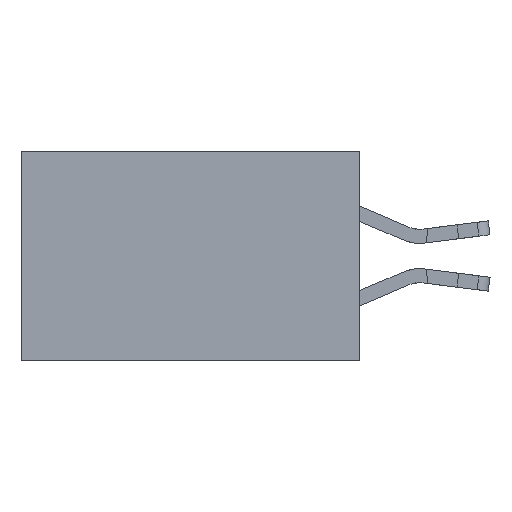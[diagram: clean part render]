
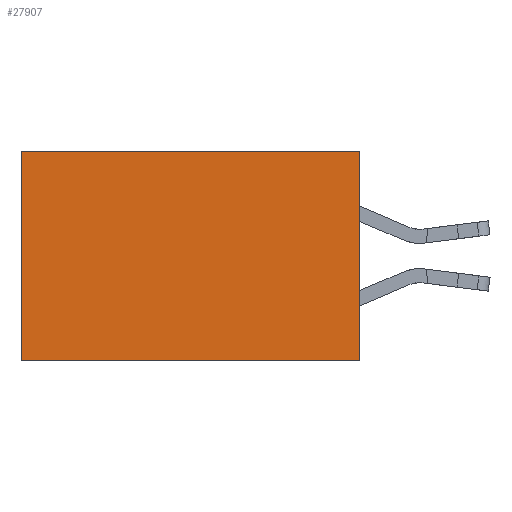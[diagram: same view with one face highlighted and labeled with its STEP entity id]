
A CAD part, left-side view. The second image highlights one B-rep face of the part: STEP entity #27907.
In plain terms, the highlighted planar face has unit normal (-1, 0, 0).
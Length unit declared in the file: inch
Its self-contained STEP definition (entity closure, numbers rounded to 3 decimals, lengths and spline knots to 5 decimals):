
#1503 = LINE ( 'NONE', #11780, #20072 ) ;
#2310 = DIRECTION ( 'NONE',  ( 0., 0., -1. ) ) ;
#2759 = DIRECTION ( 'NONE',  ( 0., 1., 0. ) ) ;
#4260 = EDGE_CURVE ( 'NONE', #8059, #28060, #25768, .T. ) ;
#5155 = ORIENTED_EDGE ( 'NONE', *, *, #7710, .T. ) ;
#6000 = CARTESIAN_POINT ( 'NONE',  ( 0.2875, 0., 0. ) ) ;
#6197 = PLANE ( 'NONE',  #6389 ) ;
#6389 = AXIS2_PLACEMENT_3D ( 'NONE', #13120, #17551, #21602 ) ;
#6698 = DIRECTION ( 'NONE',  ( 0., 0., -1. ) ) ;
#7710 = EDGE_CURVE ( 'NONE', #8059, #13851, #1503, .T. ) ;
#8059 = VERTEX_POINT ( 'NONE', #6000 ) ;
#10373 = ORIENTED_EDGE ( 'NONE', *, *, #21072, .T. ) ;
#10885 = VECTOR ( 'NONE', #6698, 39.37008 ) ;
#10946 = CARTESIAN_POINT ( 'NONE',  ( 0.2875, 0.6, 0. ) ) ;
#11146 = CARTESIAN_POINT ( 'NONE',  ( 0.2875, 0., 0. ) ) ;
#11780 = CARTESIAN_POINT ( 'NONE',  ( 0.2875, 0., 0. ) ) ;
#13120 = CARTESIAN_POINT ( 'NONE',  ( 0.2875, 0., 0. ) ) ;
#13851 = VERTEX_POINT ( 'NONE', #23755 ) ;
#14451 = CARTESIAN_POINT ( 'NONE',  ( 0.2875, 0.6, -0.37 ) ) ;
#14821 = ORIENTED_EDGE ( 'NONE', *, *, #17396, .F. ) ;
#15034 = EDGE_LOOP ( 'NONE', ( #10373, #14821, #21400, #5155 ) ) ;
#15618 = CARTESIAN_POINT ( 'NONE',  ( 0.2875, 0., -0.37 ) ) ;
#15732 = LINE ( 'NONE', #10946, #10885 ) ;
#16258 = VECTOR ( 'NONE', #21519, 39.37008 ) ;
#17396 = EDGE_CURVE ( 'NONE', #28060, #21988, #25520, .T. ) ;
#17551 = DIRECTION ( 'NONE',  ( 1., 0., 0. ) ) ;
#19302 = CARTESIAN_POINT ( 'NONE',  ( 0.2875, 0., -0.37 ) ) ;
#20072 = VECTOR ( 'NONE', #2759, 39.37008 ) ;
#21072 = EDGE_CURVE ( 'NONE', #13851, #21988, #15732, .T. ) ;
#21400 = ORIENTED_EDGE ( 'NONE', *, *, #4260, .F. ) ;
#21519 = DIRECTION ( 'NONE',  ( 0., 1., 0. ) ) ;
#21602 = DIRECTION ( 'NONE',  ( 0., 0., -1. ) ) ;
#21988 = VERTEX_POINT ( 'NONE', #14451 ) ;
#23755 = CARTESIAN_POINT ( 'NONE',  ( 0.2875, 0.6, 0. ) ) ;
#25520 = LINE ( 'NONE', #19302, #16258 ) ;
#25768 = LINE ( 'NONE', #11146, #27843 ) ;
#26930 = FACE_OUTER_BOUND ( 'NONE', #15034, .T. ) ;
#27843 = VECTOR ( 'NONE', #2310, 39.37008 ) ;
#27907 = ADVANCED_FACE ( 'NONE', ( #26930 ), #6197, .F. ) ;
#28060 = VERTEX_POINT ( 'NONE', #15618 ) ;
